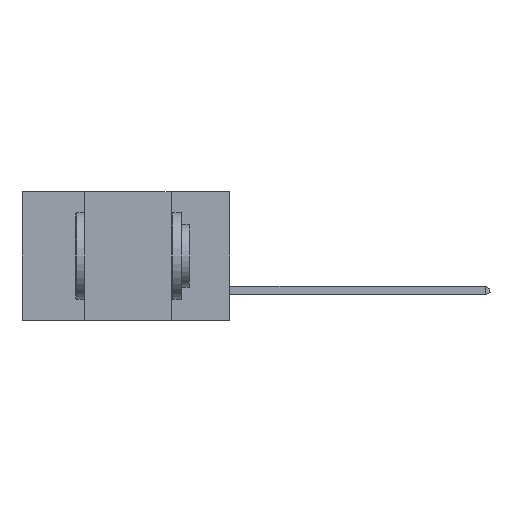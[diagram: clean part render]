
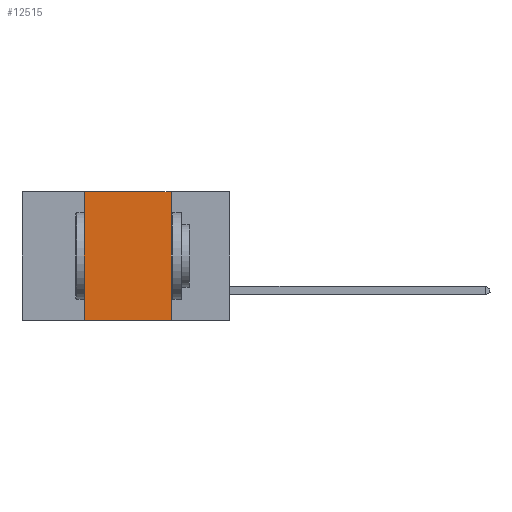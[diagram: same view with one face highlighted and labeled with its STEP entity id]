
A CAD part, left-side view. The second image highlights one B-rep face of the part: STEP entity #12515.
In plain terms, the highlighted planar face has unit normal (-1, 0, 0).
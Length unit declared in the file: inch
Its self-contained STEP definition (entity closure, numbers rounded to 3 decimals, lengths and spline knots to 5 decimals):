
#85 = FACE_OUTER_BOUND ( 'NONE', #409, .T. ) ;
#196 = CARTESIAN_POINT ( 'NONE',  ( 0., 0.17, 0. ) ) ;
#409 = EDGE_LOOP ( 'NONE', ( #19539, #29802, #6897, #29965 ) ) ;
#561 = LINE ( 'NONE', #7963, #22440 ) ;
#2787 = VERTEX_POINT ( 'NONE', #10204 ) ;
#3122 = DIRECTION ( 'NONE',  ( 0., -1., 0. ) ) ;
#5168 = CARTESIAN_POINT ( 'NONE',  ( 0., 0.42, -0.37 ) ) ;
#5253 = DIRECTION ( 'NONE',  ( 0., 0., -1. ) ) ;
#6710 = VERTEX_POINT ( 'NONE', #30109 ) ;
#6731 = VERTEX_POINT ( 'NONE', #15086 ) ;
#6897 = ORIENTED_EDGE ( 'NONE', *, *, #19029, .F. ) ;
#7028 = LINE ( 'NONE', #13664, #16222 ) ;
#7963 = CARTESIAN_POINT ( 'NONE',  ( 0., 0.6, 0. ) ) ;
#9350 = CARTESIAN_POINT ( 'NONE',  ( 0., 0.6, -0.37 ) ) ;
#10204 = CARTESIAN_POINT ( 'NONE',  ( 0., 0.17, -0.37 ) ) ;
#10627 = DIRECTION ( 'NONE',  ( 0., 0., -1. ) ) ;
#12515 = ADVANCED_FACE ( 'NONE', ( #85 ), #25349, .F. ) ;
#13664 = CARTESIAN_POINT ( 'NONE',  ( 0., 0.42, 0. ) ) ;
#15086 = CARTESIAN_POINT ( 'NONE',  ( 0., 0.17, 0. ) ) ;
#16222 = VECTOR ( 'NONE', #30837, 39.37008 ) ;
#16690 = VECTOR ( 'NONE', #5253, 39.37008 ) ;
#17848 = DIRECTION ( 'NONE',  ( 1., 0., 0. ) ) ;
#19029 = EDGE_CURVE ( 'NONE', #31701, #6710, #7028, .T. ) ;
#19539 = ORIENTED_EDGE ( 'NONE', *, *, #23959, .F. ) ;
#20291 = AXIS2_PLACEMENT_3D ( 'NONE', #25458, #17848, #10627 ) ;
#20689 = VECTOR ( 'NONE', #26537, 39.37008 ) ;
#22440 = VECTOR ( 'NONE', #3122, 39.37008 ) ;
#23599 = EDGE_CURVE ( 'NONE', #6710, #6731, #561, .T. ) ;
#23959 = EDGE_CURVE ( 'NONE', #6731, #2787, #26739, .T. ) ;
#25349 = PLANE ( 'NONE',  #20291 ) ;
#25458 = CARTESIAN_POINT ( 'NONE',  ( 0., 0.6, 0. ) ) ;
#26508 = EDGE_CURVE ( 'NONE', #31701, #2787, #27234, .T. ) ;
#26537 = DIRECTION ( 'NONE',  ( 0., -1., 0. ) ) ;
#26739 = LINE ( 'NONE', #196, #16690 ) ;
#27234 = LINE ( 'NONE', #9350, #20689 ) ;
#29802 = ORIENTED_EDGE ( 'NONE', *, *, #23599, .F. ) ;
#29965 = ORIENTED_EDGE ( 'NONE', *, *, #26508, .T. ) ;
#30109 = CARTESIAN_POINT ( 'NONE',  ( 0., 0.42, 0. ) ) ;
#30837 = DIRECTION ( 'NONE',  ( 0., 0., 1. ) ) ;
#31701 = VERTEX_POINT ( 'NONE', #5168 ) ;
